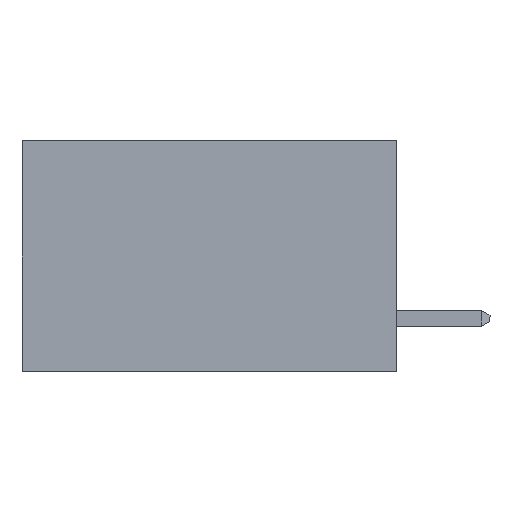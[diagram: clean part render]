
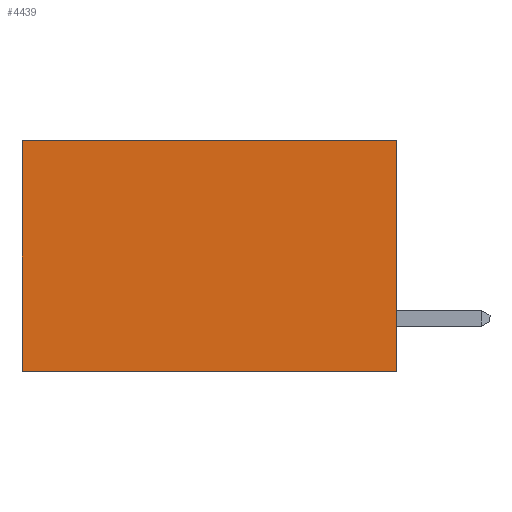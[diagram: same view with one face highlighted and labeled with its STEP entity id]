
A CAD part, left-side view. The second image highlights one B-rep face of the part: STEP entity #4439.
In plain terms, the highlighted planar face has unit normal (-1, 0, 0).
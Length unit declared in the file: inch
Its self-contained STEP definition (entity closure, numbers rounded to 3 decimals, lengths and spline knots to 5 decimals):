
#86 = VECTOR ( 'NONE', #3331, 39.37008 ) ;
#111 = FACE_OUTER_BOUND ( 'NONE', #5423, .T. ) ;
#131 = EDGE_CURVE ( 'NONE', #5730, #6001, #6596, .T. ) ;
#742 = EDGE_CURVE ( 'NONE', #3918, #809, #2663, .T. ) ;
#809 = VERTEX_POINT ( 'NONE', #6320 ) ;
#1355 = VECTOR ( 'NONE', #3214, 39.37008 ) ;
#1725 = EDGE_CURVE ( 'NONE', #5730, #3918, #3861, .T. ) ;
#2328 = EDGE_CURVE ( 'NONE', #6001, #809, #6189, .T. ) ;
#2663 = LINE ( 'NONE', #4679, #4173 ) ;
#3214 = DIRECTION ( 'NONE',  ( 0., 0., -1. ) ) ;
#3225 = CARTESIAN_POINT ( 'NONE',  ( 0.2615, 0., 0. ) ) ;
#3271 = CARTESIAN_POINT ( 'NONE',  ( 0.2615, 0.6, -0.37 ) ) ;
#3331 = DIRECTION ( 'NONE',  ( 0., 1., 0. ) ) ;
#3861 = LINE ( 'NONE', #6088, #5363 ) ;
#3918 = VERTEX_POINT ( 'NONE', #7740 ) ;
#4017 = AXIS2_PLACEMENT_3D ( 'NONE', #4964, #4788, #4787 ) ;
#4173 = VECTOR ( 'NONE', #4356, 39.37008 ) ;
#4356 = DIRECTION ( 'NONE',  ( 0., 1., 0. ) ) ;
#4439 = ADVANCED_FACE ( 'NONE', ( #111 ), #4816, .F. ) ;
#4679 = CARTESIAN_POINT ( 'NONE',  ( 0.2615, 0., -0.37 ) ) ;
#4787 = DIRECTION ( 'NONE',  ( 0., 0., -1. ) ) ;
#4788 = DIRECTION ( 'NONE',  ( 1., 0., 0. ) ) ;
#4816 = PLANE ( 'NONE',  #4017 ) ;
#4964 = CARTESIAN_POINT ( 'NONE',  ( 0.2615, 0., -0.37 ) ) ;
#5116 = CARTESIAN_POINT ( 'NONE',  ( 0.2615, 0.6, 0. ) ) ;
#5166 = ORIENTED_EDGE ( 'NONE', *, *, #742, .F. ) ;
#5363 = VECTOR ( 'NONE', #6190, 39.37008 ) ;
#5423 = EDGE_LOOP ( 'NONE', ( #7597, #5166, #7573, #6004 ) ) ;
#5730 = VERTEX_POINT ( 'NONE', #6988 ) ;
#6001 = VERTEX_POINT ( 'NONE', #5116 ) ;
#6004 = ORIENTED_EDGE ( 'NONE', *, *, #131, .T. ) ;
#6088 = CARTESIAN_POINT ( 'NONE',  ( 0.2615, 0., -0.37 ) ) ;
#6189 = LINE ( 'NONE', #3271, #1355 ) ;
#6190 = DIRECTION ( 'NONE',  ( 0., 0., -1. ) ) ;
#6320 = CARTESIAN_POINT ( 'NONE',  ( 0.2615, 0.6, -0.37 ) ) ;
#6596 = LINE ( 'NONE', #3225, #86 ) ;
#6988 = CARTESIAN_POINT ( 'NONE',  ( 0.2615, 0., 0. ) ) ;
#7573 = ORIENTED_EDGE ( 'NONE', *, *, #1725, .F. ) ;
#7597 = ORIENTED_EDGE ( 'NONE', *, *, #2328, .T. ) ;
#7740 = CARTESIAN_POINT ( 'NONE',  ( 0.2615, 0., -0.37 ) ) ;
